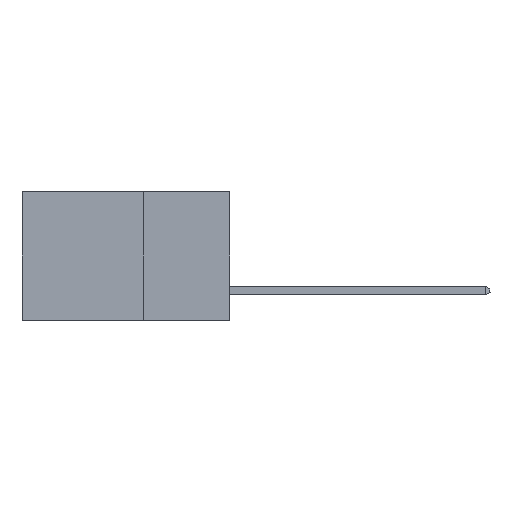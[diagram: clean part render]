
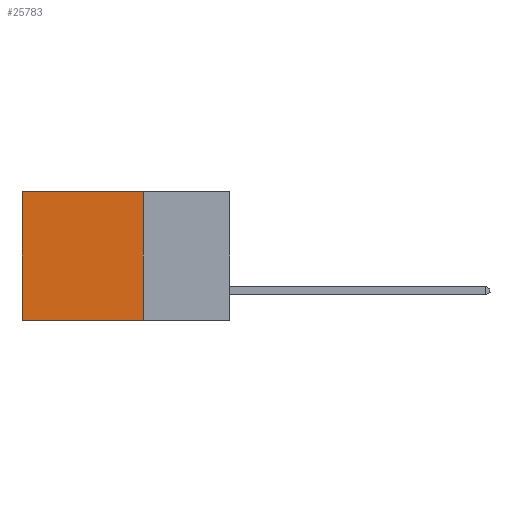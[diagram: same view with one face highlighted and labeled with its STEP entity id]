
A CAD part, left-side view. The second image highlights one B-rep face of the part: STEP entity #25783.
In plain terms, the highlighted planar face has unit normal (-1, 0, 0).
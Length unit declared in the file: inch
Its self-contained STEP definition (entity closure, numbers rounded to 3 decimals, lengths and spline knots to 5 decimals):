
#254 = VECTOR ( 'NONE', #15106, 39.37008 ) ;
#1051 = CARTESIAN_POINT ( 'NONE',  ( 0.298, 0.25, -0.37 ) ) ;
#1096 = DIRECTION ( 'NONE',  ( 0., 0., -1. ) ) ;
#1530 = DIRECTION ( 'NONE',  ( 0., 0., -1. ) ) ;
#1985 = EDGE_CURVE ( 'NONE', #25361, #7403, #21335, .T. ) ;
#2260 = VERTEX_POINT ( 'NONE', #19765 ) ;
#2918 = DIRECTION ( 'NONE',  ( 1., 0., 0. ) ) ;
#3338 = ORIENTED_EDGE ( 'NONE', *, *, #1985, .F. ) ;
#5281 = VECTOR ( 'NONE', #1530, 39.37008 ) ;
#5543 = AXIS2_PLACEMENT_3D ( 'NONE', #21644, #2918, #14821 ) ;
#6653 = ORIENTED_EDGE ( 'NONE', *, *, #29400, .T. ) ;
#7403 = VERTEX_POINT ( 'NONE', #16960 ) ;
#8571 = CARTESIAN_POINT ( 'NONE',  ( 0.298, 0.25, -0.37 ) ) ;
#9978 = PLANE ( 'NONE',  #5543 ) ;
#11290 = ORIENTED_EDGE ( 'NONE', *, *, #29022, .F. ) ;
#14775 = FACE_OUTER_BOUND ( 'NONE', #22814, .T. ) ;
#14821 = DIRECTION ( 'NONE',  ( 0., 0., -1. ) ) ;
#15106 = DIRECTION ( 'NONE',  ( 0., 1., 0. ) ) ;
#15266 = CARTESIAN_POINT ( 'NONE',  ( 0.298, 0.25, 0. ) ) ;
#16960 = CARTESIAN_POINT ( 'NONE',  ( 0.298, 0.6, -0.37 ) ) ;
#17848 = CARTESIAN_POINT ( 'NONE',  ( 0.298, 0.6, 0. ) ) ;
#19309 = LINE ( 'NONE', #24962, #25526 ) ;
#19765 = CARTESIAN_POINT ( 'NONE',  ( 0.298, 0.25, 0. ) ) ;
#20685 = VERTEX_POINT ( 'NONE', #17848 ) ;
#21335 = LINE ( 'NONE', #1051, #254 ) ;
#21644 = CARTESIAN_POINT ( 'NONE',  ( 0.298, 0.25, 0. ) ) ;
#21929 = VECTOR ( 'NONE', #1096, 39.37008 ) ;
#22814 = EDGE_LOOP ( 'NONE', ( #24710, #3338, #11290, #6653 ) ) ;
#23984 = EDGE_CURVE ( 'NONE', #20685, #7403, #25569, .T. ) ;
#24485 = LINE ( 'NONE', #15266, #21929 ) ;
#24710 = ORIENTED_EDGE ( 'NONE', *, *, #23984, .T. ) ;
#24962 = CARTESIAN_POINT ( 'NONE',  ( 0.298, 0.25, 0. ) ) ;
#25361 = VERTEX_POINT ( 'NONE', #8571 ) ;
#25526 = VECTOR ( 'NONE', #27301, 39.37008 ) ;
#25569 = LINE ( 'NONE', #29732, #5281 ) ;
#25783 = ADVANCED_FACE ( 'NONE', ( #14775 ), #9978, .F. ) ;
#27301 = DIRECTION ( 'NONE',  ( 0., 1., 0. ) ) ;
#29022 = EDGE_CURVE ( 'NONE', #2260, #25361, #24485, .T. ) ;
#29400 = EDGE_CURVE ( 'NONE', #2260, #20685, #19309, .T. ) ;
#29732 = CARTESIAN_POINT ( 'NONE',  ( 0.298, 0.6, 0. ) ) ;
